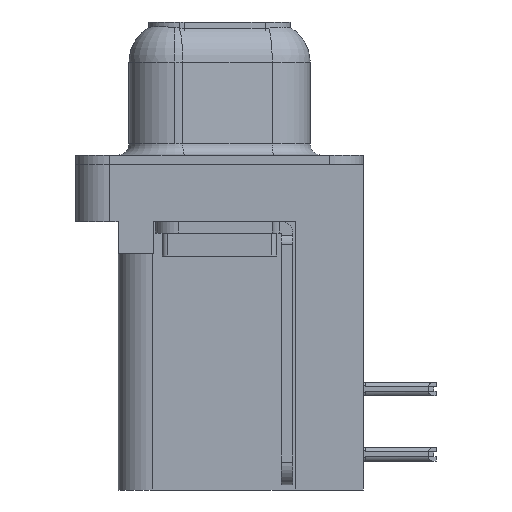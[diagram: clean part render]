
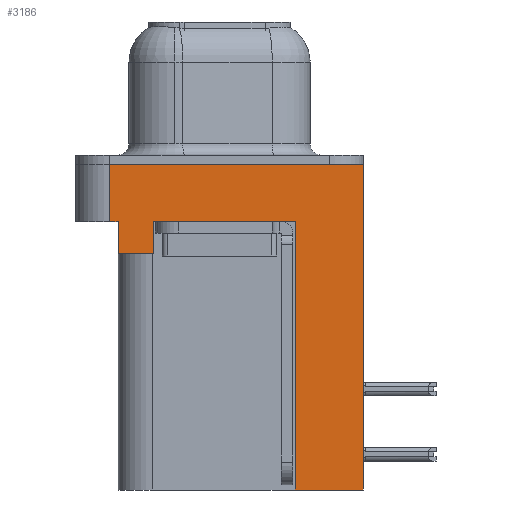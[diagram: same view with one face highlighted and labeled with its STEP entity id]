
A CAD part, left-side view. The second image highlights one B-rep face of the part: STEP entity #3186.
In plain terms, the highlighted planar face has unit normal (-1, 0, 0).
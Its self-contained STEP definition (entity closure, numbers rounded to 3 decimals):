
#91 = DIRECTION ( 'NONE',  ( 0., 0., 1. ) ) ;
#117 = EDGE_CURVE ( 'NONE', #17407, #21920, #19421, .T. ) ;
#119 = DIRECTION ( 'NONE',  ( 0., 0., 1. ) ) ;
#527 = CARTESIAN_POINT ( 'NONE',  ( -2.935, 4.775, -2.5 ) ) ;
#794 = VERTEX_POINT ( 'NONE', #11504 ) ;
#1481 = VERTEX_POINT ( 'NONE', #2254 ) ;
#1589 = CARTESIAN_POINT ( 'NONE',  ( -2.935, -3.295, -14.2 ) ) ;
#1650 = EDGE_CURVE ( 'NONE', #794, #22732, #5170, .T. ) ;
#1916 = LINE ( 'NONE', #9407, #11848 ) ;
#2234 = VERTEX_POINT ( 'NONE', #5329 ) ;
#2254 = CARTESIAN_POINT ( 'NONE',  ( -2.935, 4.425, -2.5 ) ) ;
#2333 = EDGE_LOOP ( 'NONE', ( #22655, #20283, #22262, #19405, #20433, #11673, #13008, #13715, #10135, #22619 ) ) ;
#2934 = CARTESIAN_POINT ( 'NONE',  ( -2.935, -6.275, -2.5 ) ) ;
#3186 = ADVANCED_FACE ( 'NONE', ( #11389 ), #14681, .T. ) ;
#3259 = CARTESIAN_POINT ( 'NONE',  ( -2.935, -3.295, -14.2 ) ) ;
#3303 = EDGE_CURVE ( 'NONE', #20844, #2234, #9552, .T. ) ;
#3435 = CARTESIAN_POINT ( 'NONE',  ( -2.935, -6.275, -2.5 ) ) ;
#3591 = VECTOR ( 'NONE', #22248, 1000. ) ;
#3666 = DIRECTION ( 'NONE',  ( -1., 0., 0. ) ) ;
#3938 = DIRECTION ( 'NONE',  ( 0., 0., 1. ) ) ;
#4234 = CARTESIAN_POINT ( 'NONE',  ( -2.935, 4.425, -3.9 ) ) ;
#4922 = VECTOR ( 'NONE', #21308, 1000. ) ;
#5170 = LINE ( 'NONE', #12645, #9486 ) ;
#5329 = CARTESIAN_POINT ( 'NONE',  ( -2.935, -6.275, 0. ) ) ;
#6035 = LINE ( 'NONE', #20715, #13372 ) ;
#6066 = DIRECTION ( 'NONE',  ( 0., 0., 1. ) ) ;
#6678 = EDGE_CURVE ( 'NONE', #16352, #9228, #14766, .T. ) ;
#7354 = LINE ( 'NONE', #1589, #10656 ) ;
#7791 = VECTOR ( 'NONE', #23212, 1000. ) ;
#8955 = DIRECTION ( 'NONE',  ( 0., 1., 0. ) ) ;
#9228 = VERTEX_POINT ( 'NONE', #4234 ) ;
#9377 = LINE ( 'NONE', #15354, #18492 ) ;
#9407 = CARTESIAN_POINT ( 'NONE',  ( -2.935, 2.895, -3.9 ) ) ;
#9486 = VECTOR ( 'NONE', #17782, 1000. ) ;
#9552 = LINE ( 'NONE', #3435, #17181 ) ;
#10135 = ORIENTED_EDGE ( 'NONE', *, *, #13056, .F. ) ;
#10288 = LINE ( 'NONE', #2934, #4922 ) ;
#10656 = VECTOR ( 'NONE', #8955, 1000. ) ;
#10903 = EDGE_CURVE ( 'NONE', #12023, #22732, #6035, .T. ) ;
#11389 = FACE_OUTER_BOUND ( 'NONE', #2333, .T. ) ;
#11504 = CARTESIAN_POINT ( 'NONE',  ( -2.935, 2.895, -2.5 ) ) ;
#11673 = ORIENTED_EDGE ( 'NONE', *, *, #13716, .T. ) ;
#11848 = VECTOR ( 'NONE', #91, 1000. ) ;
#12023 = VERTEX_POINT ( 'NONE', #3259 ) ;
#12136 = EDGE_CURVE ( 'NONE', #9228, #1481, #9377, .T. ) ;
#12610 = LINE ( 'NONE', #18598, #19100 ) ;
#12645 = CARTESIAN_POINT ( 'NONE',  ( -2.935, -6.275, -2.5 ) ) ;
#13008 = ORIENTED_EDGE ( 'NONE', *, *, #1650, .T. ) ;
#13056 = EDGE_CURVE ( 'NONE', #20844, #12023, #7354, .T. ) ;
#13061 = CARTESIAN_POINT ( 'NONE',  ( -2.935, 4.425, -3.9 ) ) ;
#13372 = VECTOR ( 'NONE', #3938, 1000. ) ;
#13715 = ORIENTED_EDGE ( 'NONE', *, *, #10903, .F. ) ;
#13716 = EDGE_CURVE ( 'NONE', #16352, #794, #1916, .T. ) ;
#14434 = DIRECTION ( 'NONE',  ( 0., -1., 0. ) ) ;
#14681 = PLANE ( 'NONE',  #22280 ) ;
#14766 = LINE ( 'NONE', #13061, #3591 ) ;
#15354 = CARTESIAN_POINT ( 'NONE',  ( -2.935, 4.425, -3.9 ) ) ;
#16090 = CARTESIAN_POINT ( 'NONE',  ( -2.935, -3.295, -2.5 ) ) ;
#16352 = VERTEX_POINT ( 'NONE', #20069 ) ;
#16515 = DIRECTION ( 'NONE',  ( 0., 0., 1. ) ) ;
#17181 = VECTOR ( 'NONE', #16515, 1000. ) ;
#17407 = VERTEX_POINT ( 'NONE', #527 ) ;
#17565 = CARTESIAN_POINT ( 'NONE',  ( -2.935, 4.775, -2.5 ) ) ;
#17782 = DIRECTION ( 'NONE',  ( 0., -1., 0. ) ) ;
#18492 = VECTOR ( 'NONE', #6066, 1000. ) ;
#18598 = CARTESIAN_POINT ( 'NONE',  ( -2.935, -6.275, 0. ) ) ;
#18611 = CARTESIAN_POINT ( 'NONE',  ( -2.935, -6.275, -2.5 ) ) ;
#19100 = VECTOR ( 'NONE', #14434, 1000. ) ;
#19405 = ORIENTED_EDGE ( 'NONE', *, *, #12136, .F. ) ;
#19421 = LINE ( 'NONE', #17565, #7791 ) ;
#19969 = CARTESIAN_POINT ( 'NONE',  ( -2.935, 4.775, 0. ) ) ;
#20069 = CARTESIAN_POINT ( 'NONE',  ( -2.935, 2.895, -3.9 ) ) ;
#20283 = ORIENTED_EDGE ( 'NONE', *, *, #117, .F. ) ;
#20433 = ORIENTED_EDGE ( 'NONE', *, *, #6678, .F. ) ;
#20715 = CARTESIAN_POINT ( 'NONE',  ( -2.935, -3.295, -14.2 ) ) ;
#20795 = EDGE_CURVE ( 'NONE', #21920, #2234, #12610, .T. ) ;
#20844 = VERTEX_POINT ( 'NONE', #22392 ) ;
#21308 = DIRECTION ( 'NONE',  ( 0., -1., 0. ) ) ;
#21920 = VERTEX_POINT ( 'NONE', #19969 ) ;
#22248 = DIRECTION ( 'NONE',  ( 0., 1., 0. ) ) ;
#22262 = ORIENTED_EDGE ( 'NONE', *, *, #23590, .T. ) ;
#22280 = AXIS2_PLACEMENT_3D ( 'NONE', #18611, #3666, #119 ) ;
#22392 = CARTESIAN_POINT ( 'NONE',  ( -2.935, -6.275, -14.2 ) ) ;
#22619 = ORIENTED_EDGE ( 'NONE', *, *, #3303, .T. ) ;
#22655 = ORIENTED_EDGE ( 'NONE', *, *, #20795, .F. ) ;
#22732 = VERTEX_POINT ( 'NONE', #16090 ) ;
#23212 = DIRECTION ( 'NONE',  ( 0., 0., 1. ) ) ;
#23590 = EDGE_CURVE ( 'NONE', #17407, #1481, #10288, .T. ) ;
